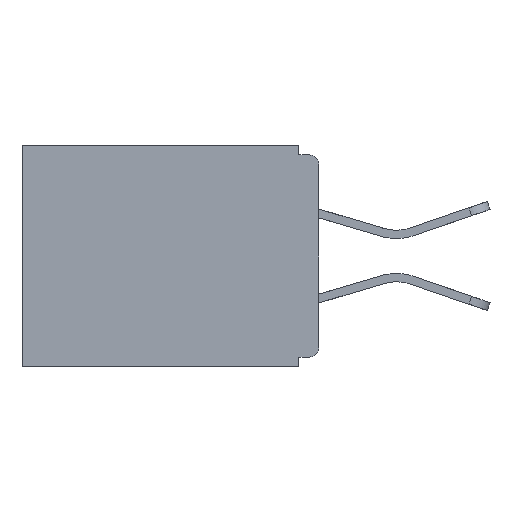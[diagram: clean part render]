
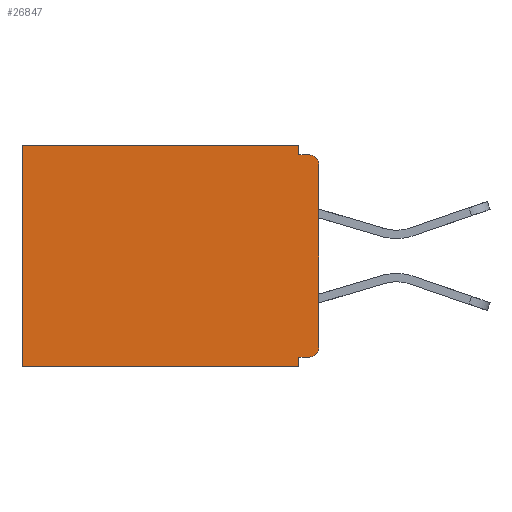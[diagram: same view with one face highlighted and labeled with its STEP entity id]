
A CAD part, left-side view. The second image highlights one B-rep face of the part: STEP entity #26847.
In plain terms, the highlighted planar face has unit normal (-1, 0, 0).
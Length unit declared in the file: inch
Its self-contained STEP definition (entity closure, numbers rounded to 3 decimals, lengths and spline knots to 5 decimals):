
#209 = DIRECTION ( 'NONE',  ( 0., -1., 0. ) ) ;
#473 = VERTEX_POINT ( 'NONE', #11741 ) ;
#474 = VECTOR ( 'NONE', #26388, 39.37008 ) ;
#931 = VERTEX_POINT ( 'NONE', #16255 ) ;
#986 = PLANE ( 'NONE',  #1729 ) ;
#1369 = VERTEX_POINT ( 'NONE', #12813 ) ;
#1386 = DIRECTION ( 'NONE',  ( 0., 1., 0. ) ) ;
#1729 = AXIS2_PLACEMENT_3D ( 'NONE', #14181, #21007, #25314 ) ;
#2247 = DIRECTION ( 'NONE',  ( 0., 0., -1. ) ) ;
#2689 = LINE ( 'NONE', #3925, #11304 ) ;
#2698 = CARTESIAN_POINT ( 'NONE',  ( 0.298, 0.015, -0.015 ) ) ;
#3025 = EDGE_LOOP ( 'NONE', ( #25611, #11512, #24790, #7968, #18186, #3719, #14737, #13678, #14847, #11432 ) ) ;
#3153 = DIRECTION ( 'NONE',  ( -1., 0., 0. ) ) ;
#3307 = VECTOR ( 'NONE', #5173, 39.37008 ) ;
#3476 = VERTEX_POINT ( 'NONE', #24785 ) ;
#3586 = EDGE_CURVE ( 'NONE', #931, #7459, #19108, .T. ) ;
#3719 = ORIENTED_EDGE ( 'NONE', *, *, #12429, .F. ) ;
#3925 = CARTESIAN_POINT ( 'NONE',  ( 0.298, 0.031, -0.343 ) ) ;
#4236 = VECTOR ( 'NONE', #2247, 39.37008 ) ;
#4253 = CARTESIAN_POINT ( 'NONE',  ( 0.298, 0.031, -0.343 ) ) ;
#5173 = DIRECTION ( 'NONE',  ( 0., 0., -1. ) ) ;
#6436 = CARTESIAN_POINT ( 'NONE',  ( 0.298, 0.031, -0.015 ) ) ;
#6582 = VERTEX_POINT ( 'NONE', #15075 ) ;
#6811 = CARTESIAN_POINT ( 'NONE',  ( 0.298, 0., -0.313 ) ) ;
#7459 = VERTEX_POINT ( 'NONE', #6811 ) ;
#7724 = DIRECTION ( 'NONE',  ( 0., 1., 0. ) ) ;
#7968 = ORIENTED_EDGE ( 'NONE', *, *, #11308, .T. ) ;
#8352 = EDGE_CURVE ( 'NONE', #473, #7459, #9383, .T. ) ;
#8464 = VECTOR ( 'NONE', #209, 39.37008 ) ;
#8837 = AXIS2_PLACEMENT_3D ( 'NONE', #16375, #3153, #18606 ) ;
#9383 = LINE ( 'NONE', #17775, #4236 ) ;
#9443 = CIRCLE ( 'NONE', #8837, 0.015 ) ;
#10200 = LINE ( 'NONE', #18392, #3307 ) ;
#11304 = VECTOR ( 'NONE', #23763, 39.37008 ) ;
#11308 = EDGE_CURVE ( 'NONE', #1369, #6582, #25375, .T. ) ;
#11432 = ORIENTED_EDGE ( 'NONE', *, *, #8352, .F. ) ;
#11512 = ORIENTED_EDGE ( 'NONE', *, *, #20673, .F. ) ;
#11611 = EDGE_CURVE ( 'NONE', #6582, #27025, #10200, .T. ) ;
#11741 = CARTESIAN_POINT ( 'NONE',  ( 0.298, 0., -0.03 ) ) ;
#11813 = LINE ( 'NONE', #16339, #13532 ) ;
#11867 = DIRECTION ( 'NONE',  ( 0., 1., 0. ) ) ;
#12429 = EDGE_CURVE ( 'NONE', #3476, #27025, #22913, .T. ) ;
#12813 = CARTESIAN_POINT ( 'NONE',  ( 0.298, 0.031, 0. ) ) ;
#13245 = EDGE_CURVE ( 'NONE', #16748, #3476, #14940, .T. ) ;
#13532 = VECTOR ( 'NONE', #1386, 39.37008 ) ;
#13678 = ORIENTED_EDGE ( 'NONE', *, *, #16889, .F. ) ;
#14181 = CARTESIAN_POINT ( 'NONE',  ( 0.298, 0., 0. ) ) ;
#14343 = LINE ( 'NONE', #22337, #8464 ) ;
#14409 = DIRECTION ( 'NONE',  ( -1., 0., 0. ) ) ;
#14605 = CARTESIAN_POINT ( 'NONE',  ( 0.298, 0.015, -0.313 ) ) ;
#14737 = ORIENTED_EDGE ( 'NONE', *, *, #13245, .F. ) ;
#14847 = ORIENTED_EDGE ( 'NONE', *, *, #3586, .T. ) ;
#14940 = LINE ( 'NONE', #4253, #474 ) ;
#15075 = CARTESIAN_POINT ( 'NONE',  ( 0.298, 0.46, 0. ) ) ;
#15752 = VECTOR ( 'NONE', #7724, 39.37008 ) ;
#16211 = CARTESIAN_POINT ( 'NONE',  ( 0.298, 0., -0.343 ) ) ;
#16255 = CARTESIAN_POINT ( 'NONE',  ( 0.298, 0.015, -0.328 ) ) ;
#16339 = CARTESIAN_POINT ( 'NONE',  ( 0.298, 0., -0.328 ) ) ;
#16375 = CARTESIAN_POINT ( 'NONE',  ( 0.298, 0.015, -0.03 ) ) ;
#16748 = VERTEX_POINT ( 'NONE', #24806 ) ;
#16889 = EDGE_CURVE ( 'NONE', #931, #16748, #11813, .T. ) ;
#17775 = CARTESIAN_POINT ( 'NONE',  ( 0.298, 0., 0. ) ) ;
#18186 = ORIENTED_EDGE ( 'NONE', *, *, #11611, .T. ) ;
#18392 = CARTESIAN_POINT ( 'NONE',  ( 0.298, 0.46, 0. ) ) ;
#18606 = DIRECTION ( 'NONE',  ( 0., 0., -1. ) ) ;
#19108 = CIRCLE ( 'NONE', #27218, 0.015 ) ;
#19268 = EDGE_CURVE ( 'NONE', #1369, #21175, #2689, .T. ) ;
#19296 = FACE_OUTER_BOUND ( 'NONE', #3025, .T. ) ;
#20673 = EDGE_CURVE ( 'NONE', #21175, #26772, #14343, .T. ) ;
#21007 = DIRECTION ( 'NONE',  ( 1., 0., 0. ) ) ;
#21175 = VERTEX_POINT ( 'NONE', #6436 ) ;
#21195 = VECTOR ( 'NONE', #11867, 39.37008 ) ;
#21324 = EDGE_CURVE ( 'NONE', #473, #26772, #9443, .T. ) ;
#22337 = CARTESIAN_POINT ( 'NONE',  ( 0.298, 0., -0.015 ) ) ;
#22913 = LINE ( 'NONE', #16211, #21195 ) ;
#23763 = DIRECTION ( 'NONE',  ( 0., 0., -1. ) ) ;
#24753 = CARTESIAN_POINT ( 'NONE',  ( 0.298, 0., 0. ) ) ;
#24785 = CARTESIAN_POINT ( 'NONE',  ( 0.298, 0.031, -0.343 ) ) ;
#24790 = ORIENTED_EDGE ( 'NONE', *, *, #19268, .F. ) ;
#24806 = CARTESIAN_POINT ( 'NONE',  ( 0.298, 0.031, -0.328 ) ) ;
#25270 = DIRECTION ( 'NONE',  ( 0., 0., -1. ) ) ;
#25314 = DIRECTION ( 'NONE',  ( 0., 0., -1. ) ) ;
#25375 = LINE ( 'NONE', #24753, #15752 ) ;
#25611 = ORIENTED_EDGE ( 'NONE', *, *, #21324, .T. ) ;
#26388 = DIRECTION ( 'NONE',  ( 0., 0., -1. ) ) ;
#26772 = VERTEX_POINT ( 'NONE', #2698 ) ;
#26847 = ADVANCED_FACE ( 'NONE', ( #19296 ), #986, .F. ) ;
#27025 = VERTEX_POINT ( 'NONE', #27932 ) ;
#27218 = AXIS2_PLACEMENT_3D ( 'NONE', #14605, #14409, #25270 ) ;
#27932 = CARTESIAN_POINT ( 'NONE',  ( 0.298, 0.46, -0.343 ) ) ;
